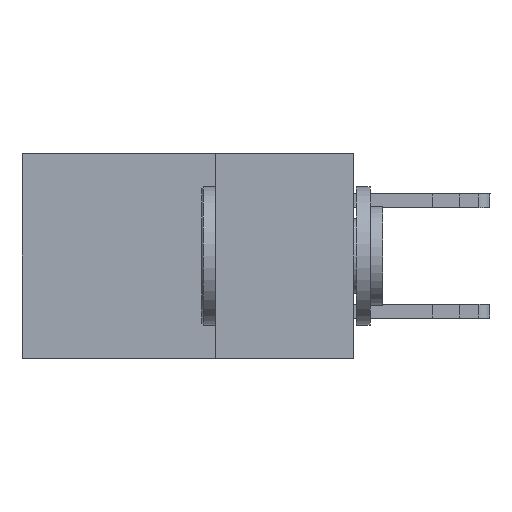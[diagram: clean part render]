
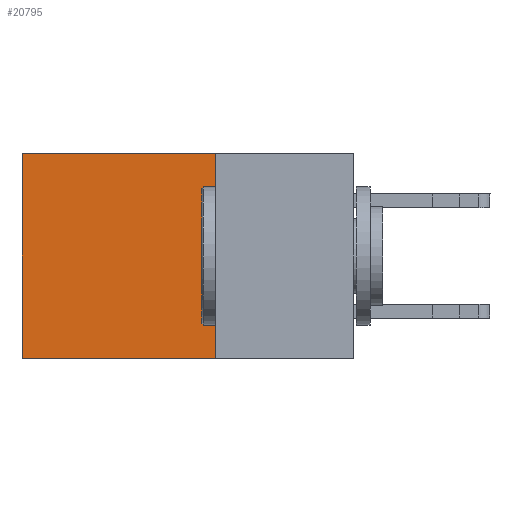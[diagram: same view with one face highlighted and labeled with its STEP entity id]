
A CAD part, left-side view. The second image highlights one B-rep face of the part: STEP entity #20795.
In plain terms, the highlighted planar face has unit normal (-1, 0, 0).
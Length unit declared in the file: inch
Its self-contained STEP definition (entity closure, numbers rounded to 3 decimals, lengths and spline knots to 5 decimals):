
#108 = DIRECTION ( 'NONE',  ( 0., 1., 0. ) ) ;
#153 = DIRECTION ( 'NONE',  ( 0., 0., -1. ) ) ;
#244 = PLANE ( 'NONE',  #4231 ) ;
#276 = VECTOR ( 'NONE', #30814, 39.37008 ) ;
#576 = LINE ( 'NONE', #7211, #2825 ) ;
#1520 = EDGE_CURVE ( 'NONE', #10247, #13327, #4243, .T. ) ;
#2220 = EDGE_CURVE ( 'NONE', #13327, #6030, #26710, .T. ) ;
#2825 = VECTOR ( 'NONE', #108, 39.37008 ) ;
#3837 = FACE_OUTER_BOUND ( 'NONE', #26006, .T. ) ;
#4231 = AXIS2_PLACEMENT_3D ( 'NONE', #5059, #4683, #153 ) ;
#4243 = LINE ( 'NONE', #28900, #24009 ) ;
#4683 = DIRECTION ( 'NONE',  ( 1., 0., 0. ) ) ;
#4877 = CARTESIAN_POINT ( 'NONE',  ( 0.2875, 0.25, -0.37 ) ) ;
#5059 = CARTESIAN_POINT ( 'NONE',  ( 0.2875, 0.25, 0. ) ) ;
#5068 = CARTESIAN_POINT ( 'NONE',  ( 0.2875, 0.25, 0. ) ) ;
#5307 = DIRECTION ( 'NONE',  ( 0., 1., 0. ) ) ;
#5308 = ORIENTED_EDGE ( 'NONE', *, *, #17172, .F. ) ;
#6030 = VERTEX_POINT ( 'NONE', #10874 ) ;
#6623 = ORIENTED_EDGE ( 'NONE', *, *, #1520, .T. ) ;
#6652 = LINE ( 'NONE', #6662, #276 ) ;
#6662 = CARTESIAN_POINT ( 'NONE',  ( 0.2875, 0.25, 0. ) ) ;
#7211 = CARTESIAN_POINT ( 'NONE',  ( 0.2875, 0.25, -0.37 ) ) ;
#9094 = DIRECTION ( 'NONE',  ( 0., 0., -1. ) ) ;
#10247 = VERTEX_POINT ( 'NONE', #5068 ) ;
#10874 = CARTESIAN_POINT ( 'NONE',  ( 0.2875, 0.6, -0.37 ) ) ;
#13327 = VERTEX_POINT ( 'NONE', #30334 ) ;
#13817 = CARTESIAN_POINT ( 'NONE',  ( 0.2875, 0.6, 0. ) ) ;
#17172 = EDGE_CURVE ( 'NONE', #10247, #30444, #6652, .T. ) ;
#18165 = EDGE_CURVE ( 'NONE', #30444, #6030, #576, .T. ) ;
#19065 = ORIENTED_EDGE ( 'NONE', *, *, #18165, .F. ) ;
#20795 = ADVANCED_FACE ( 'NONE', ( #3837 ), #244, .F. ) ;
#21483 = VECTOR ( 'NONE', #9094, 39.37008 ) ;
#24009 = VECTOR ( 'NONE', #5307, 39.37008 ) ;
#24705 = ORIENTED_EDGE ( 'NONE', *, *, #2220, .T. ) ;
#26006 = EDGE_LOOP ( 'NONE', ( #24705, #19065, #5308, #6623 ) ) ;
#26710 = LINE ( 'NONE', #13817, #21483 ) ;
#28900 = CARTESIAN_POINT ( 'NONE',  ( 0.2875, 0.25, 0. ) ) ;
#30334 = CARTESIAN_POINT ( 'NONE',  ( 0.2875, 0.6, 0. ) ) ;
#30444 = VERTEX_POINT ( 'NONE', #4877 ) ;
#30814 = DIRECTION ( 'NONE',  ( 0., 0., -1. ) ) ;
